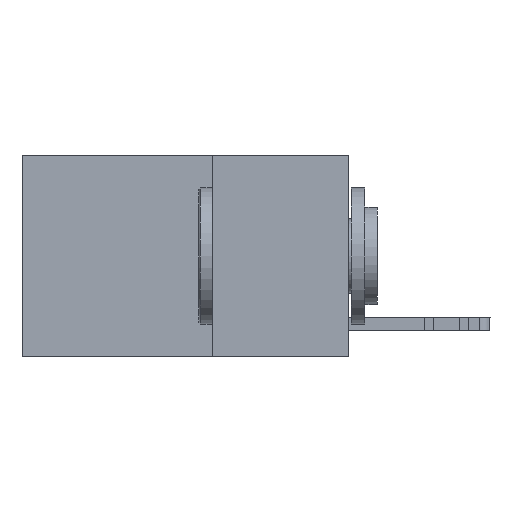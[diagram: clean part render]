
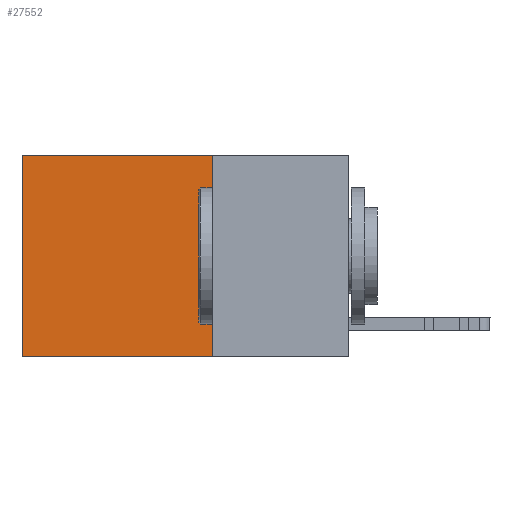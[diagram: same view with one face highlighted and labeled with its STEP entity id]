
A CAD part, left-side view. The second image highlights one B-rep face of the part: STEP entity #27552.
In plain terms, the highlighted planar face has unit normal (-1, 0, 0).
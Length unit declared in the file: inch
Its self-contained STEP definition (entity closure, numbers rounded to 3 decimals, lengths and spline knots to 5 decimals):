
#292 = DIRECTION ( 'NONE',  ( 0., 1., 0. ) ) ;
#946 = CARTESIAN_POINT ( 'NONE',  ( 0.2625, 0.25, 0. ) ) ;
#3022 = AXIS2_PLACEMENT_3D ( 'NONE', #26147, #26583, #28688 ) ;
#3995 = EDGE_LOOP ( 'NONE', ( #24674, #11213, #5362, #17910 ) ) ;
#4071 = VERTEX_POINT ( 'NONE', #15203 ) ;
#4716 = EDGE_CURVE ( 'NONE', #7891, #27005, #23793, .T. ) ;
#5362 = ORIENTED_EDGE ( 'NONE', *, *, #15548, .F. ) ;
#7790 = VECTOR ( 'NONE', #19586, 39.37008 ) ;
#7891 = VERTEX_POINT ( 'NONE', #26212 ) ;
#8353 = PLANE ( 'NONE',  #3022 ) ;
#8703 = VECTOR ( 'NONE', #23357, 39.37008 ) ;
#9151 = CARTESIAN_POINT ( 'NONE',  ( 0.2625, 0.6, 0. ) ) ;
#9175 = VECTOR ( 'NONE', #292, 39.37008 ) ;
#9788 = VECTOR ( 'NONE', #16961, 39.37008 ) ;
#11213 = ORIENTED_EDGE ( 'NONE', *, *, #26272, .F. ) ;
#13377 = EDGE_CURVE ( 'NONE', #27005, #20759, #26146, .T. ) ;
#15203 = CARTESIAN_POINT ( 'NONE',  ( 0.2625, 0.25, -0.37 ) ) ;
#15548 = EDGE_CURVE ( 'NONE', #7891, #4071, #19340, .T. ) ;
#16961 = DIRECTION ( 'NONE',  ( 0., 0., -1. ) ) ;
#17490 = FACE_OUTER_BOUND ( 'NONE', #3995, .T. ) ;
#17910 = ORIENTED_EDGE ( 'NONE', *, *, #4716, .T. ) ;
#18377 = CARTESIAN_POINT ( 'NONE',  ( 0.2625, 0.25, -0.37 ) ) ;
#18827 = CARTESIAN_POINT ( 'NONE',  ( 0.2625, 0.6, -0.37 ) ) ;
#18905 = CARTESIAN_POINT ( 'NONE',  ( 0.2625, 0.25, 0. ) ) ;
#19340 = LINE ( 'NONE', #18905, #9788 ) ;
#19586 = DIRECTION ( 'NONE',  ( 0., 0., -1. ) ) ;
#20759 = VERTEX_POINT ( 'NONE', #18827 ) ;
#21675 = CARTESIAN_POINT ( 'NONE',  ( 0.2625, 0.6, 0. ) ) ;
#23357 = DIRECTION ( 'NONE',  ( 0., 1., 0. ) ) ;
#23793 = LINE ( 'NONE', #946, #8703 ) ;
#24674 = ORIENTED_EDGE ( 'NONE', *, *, #13377, .T. ) ;
#25687 = LINE ( 'NONE', #18377, #9175 ) ;
#26146 = LINE ( 'NONE', #21675, #7790 ) ;
#26147 = CARTESIAN_POINT ( 'NONE',  ( 0.2625, 0.25, 0. ) ) ;
#26212 = CARTESIAN_POINT ( 'NONE',  ( 0.2625, 0.25, 0. ) ) ;
#26272 = EDGE_CURVE ( 'NONE', #4071, #20759, #25687, .T. ) ;
#26583 = DIRECTION ( 'NONE',  ( 1., 0., 0. ) ) ;
#27005 = VERTEX_POINT ( 'NONE', #9151 ) ;
#27552 = ADVANCED_FACE ( 'NONE', ( #17490 ), #8353, .F. ) ;
#28688 = DIRECTION ( 'NONE',  ( 0., 0., -1. ) ) ;
